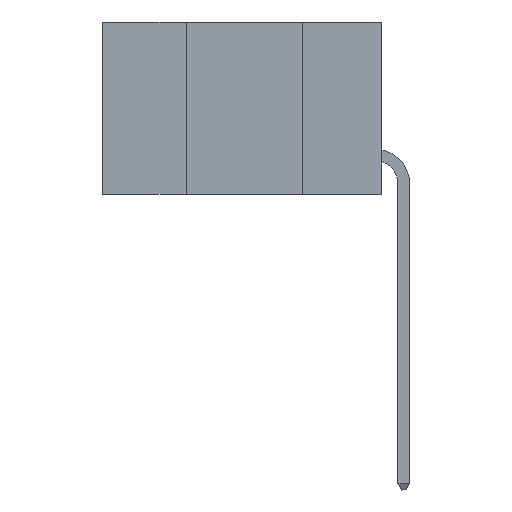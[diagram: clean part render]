
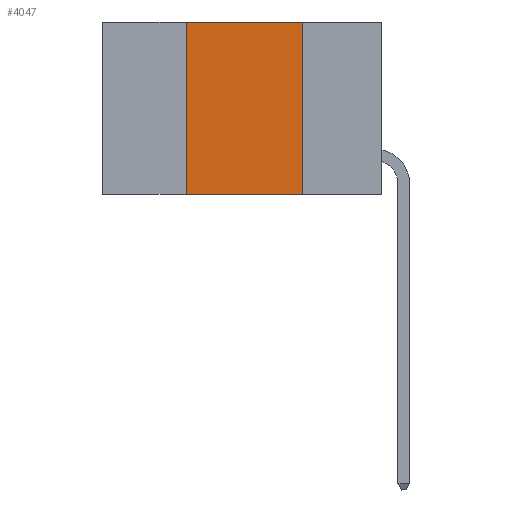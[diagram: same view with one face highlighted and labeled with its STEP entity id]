
A CAD part, left-side view. The second image highlights one B-rep face of the part: STEP entity #4047.
In plain terms, the highlighted planar face has unit normal (-1, 0, 0).
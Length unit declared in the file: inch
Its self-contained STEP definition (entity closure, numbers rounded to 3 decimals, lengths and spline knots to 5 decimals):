
#240 = ORIENTED_EDGE ( 'NONE', *, *, #7541, .F. ) ;
#769 = LINE ( 'NONE', #9572, #5313 ) ;
#884 = LINE ( 'NONE', #4083, #6116 ) ;
#961 = CARTESIAN_POINT ( 'NONE',  ( 0., 0.42, -0.37 ) ) ;
#1901 = FACE_OUTER_BOUND ( 'NONE', #7238, .T. ) ;
#2088 = AXIS2_PLACEMENT_3D ( 'NONE', #3676, #4440, #9593 ) ;
#2665 = CARTESIAN_POINT ( 'NONE',  ( 0., 0.17, 0. ) ) ;
#2721 = DIRECTION ( 'NONE',  ( 0., 0., -1. ) ) ;
#2788 = VERTEX_POINT ( 'NONE', #2925 ) ;
#2874 = ORIENTED_EDGE ( 'NONE', *, *, #3607, .T. ) ;
#2925 = CARTESIAN_POINT ( 'NONE',  ( 0., 0.17, 0. ) ) ;
#3322 = EDGE_CURVE ( 'NONE', #7002, #2788, #769, .T. ) ;
#3607 = EDGE_CURVE ( 'NONE', #7588, #5200, #884, .T. ) ;
#3676 = CARTESIAN_POINT ( 'NONE',  ( 0., 0.6, 0. ) ) ;
#4047 = ADVANCED_FACE ( 'NONE', ( #1901 ), #8104, .F. ) ;
#4083 = CARTESIAN_POINT ( 'NONE',  ( 0., 0.6, -0.37 ) ) ;
#4440 = DIRECTION ( 'NONE',  ( 1., 0., 0. ) ) ;
#4746 = EDGE_CURVE ( 'NONE', #2788, #5200, #7911, .T. ) ;
#5200 = VERTEX_POINT ( 'NONE', #6160 ) ;
#5262 = DIRECTION ( 'NONE',  ( 0., -1., 0. ) ) ;
#5313 = VECTOR ( 'NONE', #5262, 39.37008 ) ;
#6116 = VECTOR ( 'NONE', #7659, 39.37008 ) ;
#6160 = CARTESIAN_POINT ( 'NONE',  ( 0., 0.17, -0.37 ) ) ;
#6434 = LINE ( 'NONE', #8153, #8824 ) ;
#6656 = ORIENTED_EDGE ( 'NONE', *, *, #3322, .F. ) ;
#6784 = ORIENTED_EDGE ( 'NONE', *, *, #4746, .F. ) ;
#6859 = DIRECTION ( 'NONE',  ( 0., 0., 1. ) ) ;
#7002 = VERTEX_POINT ( 'NONE', #8246 ) ;
#7238 = EDGE_LOOP ( 'NONE', ( #6784, #6656, #240, #2874 ) ) ;
#7541 = EDGE_CURVE ( 'NONE', #7588, #7002, #6434, .T. ) ;
#7580 = VECTOR ( 'NONE', #2721, 39.37008 ) ;
#7588 = VERTEX_POINT ( 'NONE', #961 ) ;
#7659 = DIRECTION ( 'NONE',  ( 0., -1., 0. ) ) ;
#7911 = LINE ( 'NONE', #2665, #7580 ) ;
#8104 = PLANE ( 'NONE',  #2088 ) ;
#8153 = CARTESIAN_POINT ( 'NONE',  ( 0., 0.42, 0. ) ) ;
#8246 = CARTESIAN_POINT ( 'NONE',  ( 0., 0.42, 0. ) ) ;
#8824 = VECTOR ( 'NONE', #6859, 39.37008 ) ;
#9572 = CARTESIAN_POINT ( 'NONE',  ( 0., 0.6, 0. ) ) ;
#9593 = DIRECTION ( 'NONE',  ( 0., 0., -1. ) ) ;
